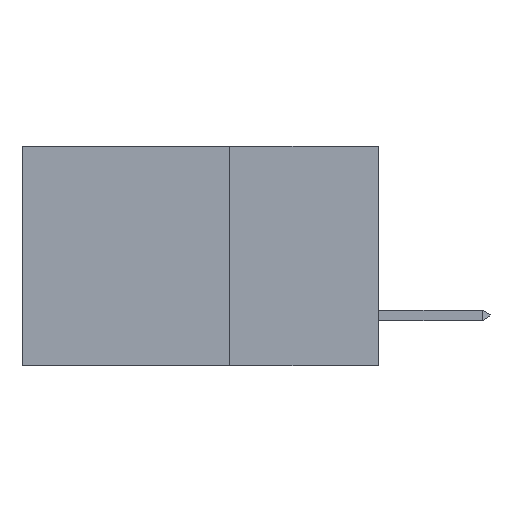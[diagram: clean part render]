
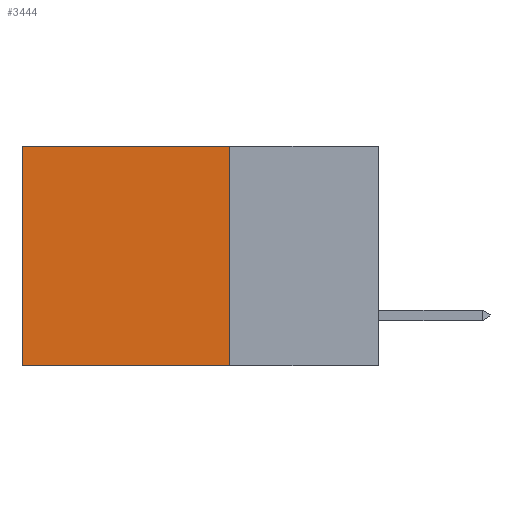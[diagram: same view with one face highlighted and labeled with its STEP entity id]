
A CAD part, left-side view. The second image highlights one B-rep face of the part: STEP entity #3444.
In plain terms, the highlighted planar face has unit normal (-1, 0, 0).
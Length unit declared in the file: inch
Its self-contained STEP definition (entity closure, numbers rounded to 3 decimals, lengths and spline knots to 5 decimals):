
#234 = CARTESIAN_POINT ( 'NONE',  ( 0.2615, 0.25, -0.37 ) ) ;
#642 = DIRECTION ( 'NONE',  ( 0., 1., 0. ) ) ;
#759 = CARTESIAN_POINT ( 'NONE',  ( 0.2615, 0.25, -0.37 ) ) ;
#954 = ORIENTED_EDGE ( 'NONE', *, *, #8800, .F. ) ;
#1191 = ORIENTED_EDGE ( 'NONE', *, *, #7469, .F. ) ;
#1466 = DIRECTION ( 'NONE',  ( 0., 1., 0. ) ) ;
#1701 = ORIENTED_EDGE ( 'NONE', *, *, #10416, .T. ) ;
#1824 = VERTEX_POINT ( 'NONE', #10164 ) ;
#2029 = VERTEX_POINT ( 'NONE', #5774 ) ;
#2390 = VECTOR ( 'NONE', #5435, 39.37008 ) ;
#3444 = ADVANCED_FACE ( 'NONE', ( #8385 ), #5334, .F. ) ;
#3978 = CARTESIAN_POINT ( 'NONE',  ( 0.2615, 0.25, -0.37 ) ) ;
#4235 = VERTEX_POINT ( 'NONE', #7593 ) ;
#4439 = ORIENTED_EDGE ( 'NONE', *, *, #8178, .T. ) ;
#5334 = PLANE ( 'NONE',  #7450 ) ;
#5435 = DIRECTION ( 'NONE',  ( 0., 0., -1. ) ) ;
#5580 = LINE ( 'NONE', #759, #6073 ) ;
#5774 = CARTESIAN_POINT ( 'NONE',  ( 0.2615, 0.6, 0. ) ) ;
#5944 = EDGE_LOOP ( 'NONE', ( #1701, #1191, #954, #4439 ) ) ;
#6073 = VECTOR ( 'NONE', #9820, 39.37008 ) ;
#6141 = DIRECTION ( 'NONE',  ( 1., 0., 0. ) ) ;
#6193 = LINE ( 'NONE', #6336, #2390 ) ;
#6336 = CARTESIAN_POINT ( 'NONE',  ( 0.2615, 0.6, -0.37 ) ) ;
#6429 = LINE ( 'NONE', #3978, #7771 ) ;
#6853 = VERTEX_POINT ( 'NONE', #6932 ) ;
#6932 = CARTESIAN_POINT ( 'NONE',  ( 0.2615, 0.25, -0.37 ) ) ;
#7450 = AXIS2_PLACEMENT_3D ( 'NONE', #234, #6141, #8604 ) ;
#7469 = EDGE_CURVE ( 'NONE', #6853, #4235, #6429, .T. ) ;
#7593 = CARTESIAN_POINT ( 'NONE',  ( 0.2615, 0.6, -0.37 ) ) ;
#7771 = VECTOR ( 'NONE', #642, 39.37008 ) ;
#7945 = VECTOR ( 'NONE', #1466, 39.37008 ) ;
#8178 = EDGE_CURVE ( 'NONE', #1824, #2029, #9518, .T. ) ;
#8385 = FACE_OUTER_BOUND ( 'NONE', #5944, .T. ) ;
#8604 = DIRECTION ( 'NONE',  ( 0., 0., -1. ) ) ;
#8800 = EDGE_CURVE ( 'NONE', #1824, #6853, #5580, .T. ) ;
#9518 = LINE ( 'NONE', #10261, #7945 ) ;
#9820 = DIRECTION ( 'NONE',  ( 0., 0., -1. ) ) ;
#10164 = CARTESIAN_POINT ( 'NONE',  ( 0.2615, 0.25, 0. ) ) ;
#10261 = CARTESIAN_POINT ( 'NONE',  ( 0.2615, 0.25, 0. ) ) ;
#10416 = EDGE_CURVE ( 'NONE', #2029, #4235, #6193, .T. ) ;
